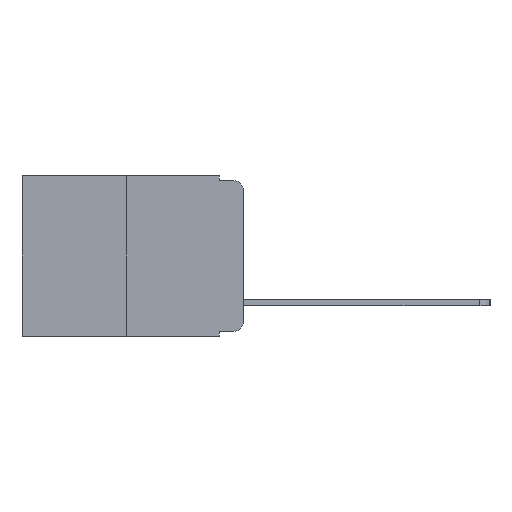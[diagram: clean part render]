
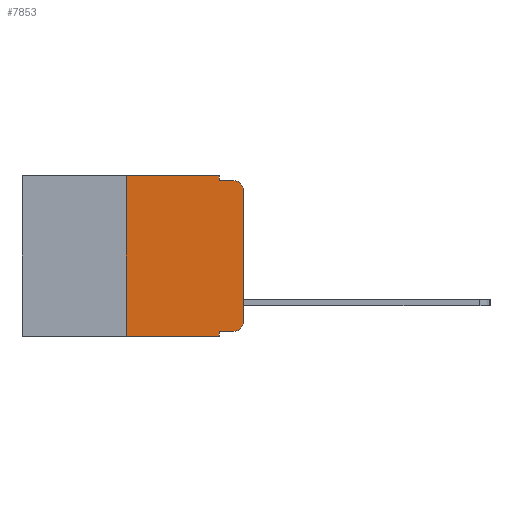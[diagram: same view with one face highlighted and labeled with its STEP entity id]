
A CAD part, left-side view. The second image highlights one B-rep face of the part: STEP entity #7853.
In plain terms, the highlighted planar face has unit normal (-1, 0, 0).
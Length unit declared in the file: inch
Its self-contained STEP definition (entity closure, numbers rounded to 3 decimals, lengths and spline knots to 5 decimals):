
#70 = DIRECTION ( 'NONE',  ( 0., 0., -1. ) ) ;
#271 = CIRCLE ( 'NONE', #8507, 0.02 ) ;
#359 = EDGE_CURVE ( 'NONE', #8891, #4185, #10124, .T. ) ;
#580 = ORIENTED_EDGE ( 'NONE', *, *, #5511, .T. ) ;
#764 = VERTEX_POINT ( 'NONE', #2071 ) ;
#1034 = EDGE_CURVE ( 'NONE', #8891, #6521, #2677, .T. ) ;
#1139 = CARTESIAN_POINT ( 'NONE',  ( 0., 0., -0.313 ) ) ;
#1229 = ORIENTED_EDGE ( 'NONE', *, *, #3002, .F. ) ;
#1590 = CARTESIAN_POINT ( 'NONE',  ( 0., 0.25, -0.343 ) ) ;
#2071 = CARTESIAN_POINT ( 'NONE',  ( 0., 0.25, 0. ) ) ;
#2094 = CARTESIAN_POINT ( 'NONE',  ( 0., 0.051, 0. ) ) ;
#2191 = LINE ( 'NONE', #8331, #11413 ) ;
#2355 = EDGE_CURVE ( 'NONE', #4956, #764, #2638, .T. ) ;
#2390 = VECTOR ( 'NONE', #11357, 39.37008 ) ;
#2454 = ORIENTED_EDGE ( 'NONE', *, *, #359, .T. ) ;
#2541 = CARTESIAN_POINT ( 'NONE',  ( 0., 0.051, -0.333 ) ) ;
#2638 = LINE ( 'NONE', #8596, #9812 ) ;
#2677 = LINE ( 'NONE', #4686, #5189 ) ;
#2725 = VECTOR ( 'NONE', #2962, 39.37008 ) ;
#2962 = DIRECTION ( 'NONE',  ( 0., 0., 1. ) ) ;
#3002 = EDGE_CURVE ( 'NONE', #10415, #11101, #2191, .T. ) ;
#3481 = VERTEX_POINT ( 'NONE', #9196 ) ;
#3607 = EDGE_CURVE ( 'NONE', #11101, #4201, #10334, .T. ) ;
#3618 = DIRECTION ( 'NONE',  ( 0., 0., 1. ) ) ;
#3726 = VECTOR ( 'NONE', #5094, 39.37008 ) ;
#3807 = DIRECTION ( 'NONE',  ( 0., -1., 0. ) ) ;
#3893 = VERTEX_POINT ( 'NONE', #1139 ) ;
#4185 = VERTEX_POINT ( 'NONE', #11716 ) ;
#4201 = VERTEX_POINT ( 'NONE', #7395 ) ;
#4360 = CARTESIAN_POINT ( 'NONE',  ( 0., 0.473, 0. ) ) ;
#4686 = CARTESIAN_POINT ( 'NONE',  ( 0., 0.051, 0. ) ) ;
#4888 = EDGE_CURVE ( 'NONE', #3481, #4201, #271, .T. ) ;
#4956 = VERTEX_POINT ( 'NONE', #1590 ) ;
#4970 = ORIENTED_EDGE ( 'NONE', *, *, #11535, .T. ) ;
#5094 = DIRECTION ( 'NONE',  ( 0., -1., 0. ) ) ;
#5189 = VECTOR ( 'NONE', #6109, 39.37008 ) ;
#5340 = DIRECTION ( 'NONE',  ( 0., 0., -1. ) ) ;
#5349 = LINE ( 'NONE', #9226, #5930 ) ;
#5511 = EDGE_CURVE ( 'NONE', #3893, #3481, #9883, .T. ) ;
#5722 = DIRECTION ( 'NONE',  ( 0., -1., 0. ) ) ;
#5730 = CARTESIAN_POINT ( 'NONE',  ( 0., 0.051, -0.01 ) ) ;
#5813 = CARTESIAN_POINT ( 'NONE',  ( 0., 0.02, -0.03 ) ) ;
#5830 = DIRECTION ( 'NONE',  ( -1., 0., 0. ) ) ;
#5831 = DIRECTION ( 'NONE',  ( -1., 0., 0. ) ) ;
#5923 = DIRECTION ( 'NONE',  ( 0., 0., -1. ) ) ;
#5930 = VECTOR ( 'NONE', #3807, 39.37008 ) ;
#5993 = ORIENTED_EDGE ( 'NONE', *, *, #3607, .F. ) ;
#6096 = CIRCLE ( 'NONE', #11763, 0.02 ) ;
#6109 = DIRECTION ( 'NONE',  ( 0., 0., -1. ) ) ;
#6268 = ORIENTED_EDGE ( 'NONE', *, *, #6756, .F. ) ;
#6322 = CARTESIAN_POINT ( 'NONE',  ( 0., 0.051, -0.343 ) ) ;
#6521 = VERTEX_POINT ( 'NONE', #6322 ) ;
#6649 = CARTESIAN_POINT ( 'NONE',  ( 0., 0., 0. ) ) ;
#6756 = EDGE_CURVE ( 'NONE', #764, #10415, #5349, .T. ) ;
#6771 = CARTESIAN_POINT ( 'NONE',  ( 0., 0.051, -0.01 ) ) ;
#7395 = CARTESIAN_POINT ( 'NONE',  ( 0., 0.02, -0.01 ) ) ;
#7472 = EDGE_LOOP ( 'NONE', ( #580, #10313, #5993, #1229, #6268, #8877, #11115, #11652, #2454, #4970 ) ) ;
#7853 = ADVANCED_FACE ( 'NONE', ( #11432 ), #11374, .F. ) ;
#8065 = VECTOR ( 'NONE', #5722, 39.37008 ) ;
#8331 = CARTESIAN_POINT ( 'NONE',  ( 0., 0.051, 0. ) ) ;
#8507 = AXIS2_PLACEMENT_3D ( 'NONE', #5813, #5830, #5923 ) ;
#8596 = CARTESIAN_POINT ( 'NONE',  ( 0., 0.25, 0. ) ) ;
#8877 = ORIENTED_EDGE ( 'NONE', *, *, #2355, .F. ) ;
#8891 = VERTEX_POINT ( 'NONE', #2541 ) ;
#9196 = CARTESIAN_POINT ( 'NONE',  ( 0., 0., -0.03 ) ) ;
#9226 = CARTESIAN_POINT ( 'NONE',  ( 0., 0.473, 0. ) ) ;
#9274 = AXIS2_PLACEMENT_3D ( 'NONE', #4360, #10545, #5340 ) ;
#9500 = CARTESIAN_POINT ( 'NONE',  ( 0., 0.473, -0.343 ) ) ;
#9812 = VECTOR ( 'NONE', #3618, 39.37008 ) ;
#9883 = LINE ( 'NONE', #6649, #2725 ) ;
#10050 = DIRECTION ( 'NONE',  ( 0., 0., -1. ) ) ;
#10124 = LINE ( 'NONE', #11223, #2390 ) ;
#10313 = ORIENTED_EDGE ( 'NONE', *, *, #4888, .T. ) ;
#10334 = LINE ( 'NONE', #5730, #8065 ) ;
#10415 = VERTEX_POINT ( 'NONE', #2094 ) ;
#10545 = DIRECTION ( 'NONE',  ( 1., 0., 0. ) ) ;
#11015 = CARTESIAN_POINT ( 'NONE',  ( 0., 0.02, -0.313 ) ) ;
#11101 = VERTEX_POINT ( 'NONE', #6771 ) ;
#11115 = ORIENTED_EDGE ( 'NONE', *, *, #11683, .T. ) ;
#11223 = CARTESIAN_POINT ( 'NONE',  ( 0., 0.051, -0.333 ) ) ;
#11342 = LINE ( 'NONE', #9500, #3726 ) ;
#11357 = DIRECTION ( 'NONE',  ( 0., -1., 0. ) ) ;
#11374 = PLANE ( 'NONE',  #9274 ) ;
#11413 = VECTOR ( 'NONE', #10050, 39.37008 ) ;
#11432 = FACE_OUTER_BOUND ( 'NONE', #7472, .T. ) ;
#11535 = EDGE_CURVE ( 'NONE', #4185, #3893, #6096, .T. ) ;
#11652 = ORIENTED_EDGE ( 'NONE', *, *, #1034, .F. ) ;
#11683 = EDGE_CURVE ( 'NONE', #4956, #6521, #11342, .T. ) ;
#11716 = CARTESIAN_POINT ( 'NONE',  ( 0., 0.02, -0.333 ) ) ;
#11763 = AXIS2_PLACEMENT_3D ( 'NONE', #11015, #5831, #70 ) ;
